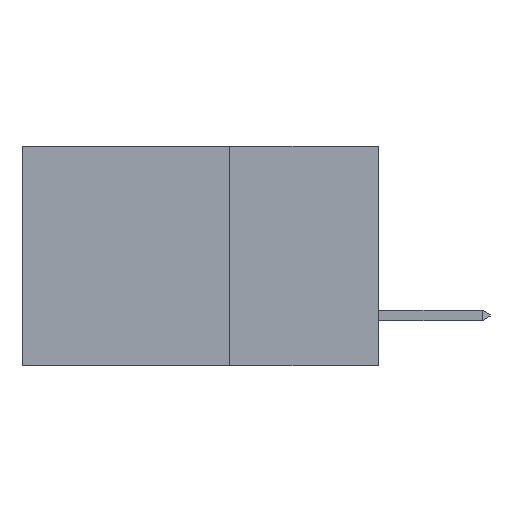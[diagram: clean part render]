
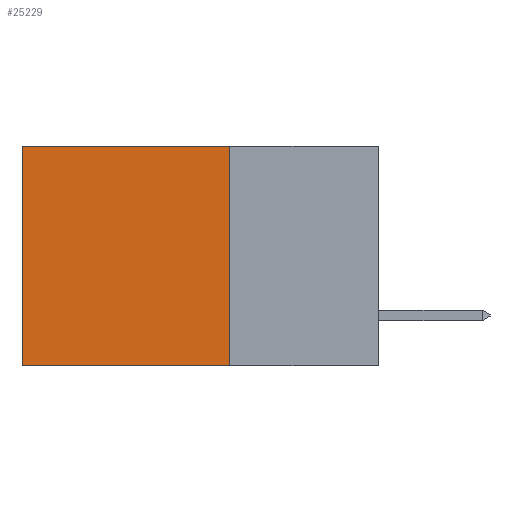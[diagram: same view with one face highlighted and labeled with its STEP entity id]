
A CAD part, left-side view. The second image highlights one B-rep face of the part: STEP entity #25229.
In plain terms, the highlighted planar face has unit normal (-1, 0, 0).
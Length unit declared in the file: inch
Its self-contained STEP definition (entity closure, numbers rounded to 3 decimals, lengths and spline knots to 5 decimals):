
#4911 = LINE ( 'NONE', #18319, #26320 ) ;
#5749 = PLANE ( 'NONE',  #13822 ) ;
#7406 = ORIENTED_EDGE ( 'NONE', *, *, #11397, .F. ) ;
#8039 = EDGE_CURVE ( 'NONE', #11566, #26877, #26738, .T. ) ;
#9387 = DIRECTION ( 'NONE',  ( 0., 1., 0. ) ) ;
#9916 = DIRECTION ( 'NONE',  ( 0., 0., -1. ) ) ;
#11397 = EDGE_CURVE ( 'NONE', #11667, #26877, #18239, .T. ) ;
#11566 = VERTEX_POINT ( 'NONE', #24816 ) ;
#11667 = VERTEX_POINT ( 'NONE', #17011 ) ;
#13160 = VERTEX_POINT ( 'NONE', #15985 ) ;
#13822 = AXIS2_PLACEMENT_3D ( 'NONE', #20344, #22423, #9916 ) ;
#13931 = EDGE_CURVE ( 'NONE', #13160, #11566, #4911, .T. ) ;
#14171 = EDGE_CURVE ( 'NONE', #13160, #11667, #17673, .T. ) ;
#14830 = CARTESIAN_POINT ( 'NONE',  ( 0.298, 0.6, 0. ) ) ;
#15623 = VECTOR ( 'NONE', #9387, 39.37008 ) ;
#15985 = CARTESIAN_POINT ( 'NONE',  ( 0.298, 0.25, 0. ) ) ;
#16330 = DIRECTION ( 'NONE',  ( 0., 1., 0. ) ) ;
#16494 = VECTOR ( 'NONE', #19029, 39.37008 ) ;
#17011 = CARTESIAN_POINT ( 'NONE',  ( 0.298, 0.25, -0.37 ) ) ;
#17178 = ORIENTED_EDGE ( 'NONE', *, *, #8039, .T. ) ;
#17673 = LINE ( 'NONE', #19111, #25979 ) ;
#17838 = CARTESIAN_POINT ( 'NONE',  ( 0.298, 0.6, -0.37 ) ) ;
#18239 = LINE ( 'NONE', #23922, #15623 ) ;
#18319 = CARTESIAN_POINT ( 'NONE',  ( 0.298, 0.25, 0. ) ) ;
#19029 = DIRECTION ( 'NONE',  ( 0., 0., -1. ) ) ;
#19111 = CARTESIAN_POINT ( 'NONE',  ( 0.298, 0.25, 0. ) ) ;
#19588 = EDGE_LOOP ( 'NONE', ( #17178, #7406, #24308, #22479 ) ) ;
#20344 = CARTESIAN_POINT ( 'NONE',  ( 0.298, 0.25, 0. ) ) ;
#21201 = DIRECTION ( 'NONE',  ( 0., 0., -1. ) ) ;
#22423 = DIRECTION ( 'NONE',  ( 1., 0., 0. ) ) ;
#22479 = ORIENTED_EDGE ( 'NONE', *, *, #13931, .T. ) ;
#23398 = FACE_OUTER_BOUND ( 'NONE', #19588, .T. ) ;
#23922 = CARTESIAN_POINT ( 'NONE',  ( 0.298, 0.25, -0.37 ) ) ;
#24308 = ORIENTED_EDGE ( 'NONE', *, *, #14171, .F. ) ;
#24816 = CARTESIAN_POINT ( 'NONE',  ( 0.298, 0.6, 0. ) ) ;
#25229 = ADVANCED_FACE ( 'NONE', ( #23398 ), #5749, .F. ) ;
#25979 = VECTOR ( 'NONE', #21201, 39.37008 ) ;
#26320 = VECTOR ( 'NONE', #16330, 39.37008 ) ;
#26738 = LINE ( 'NONE', #14830, #16494 ) ;
#26877 = VERTEX_POINT ( 'NONE', #17838 ) ;
